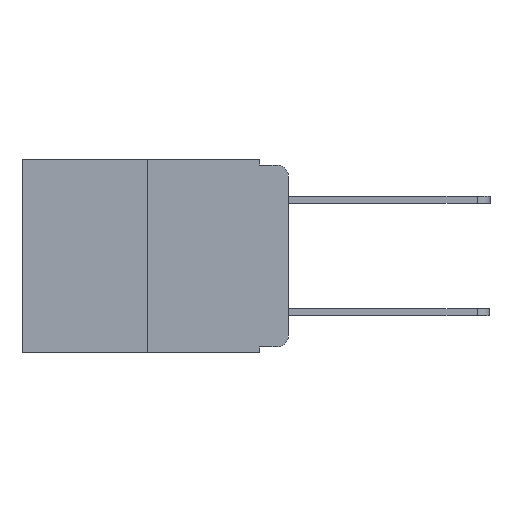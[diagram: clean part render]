
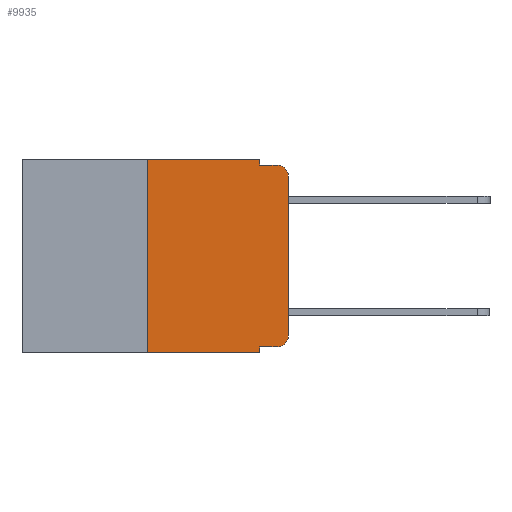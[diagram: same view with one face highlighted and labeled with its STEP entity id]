
A CAD part, left-side view. The second image highlights one B-rep face of the part: STEP entity #9935.
In plain terms, the highlighted planar face has unit normal (-1, 0, 0).
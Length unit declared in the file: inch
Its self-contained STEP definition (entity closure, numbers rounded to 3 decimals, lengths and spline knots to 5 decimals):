
#72 = DIRECTION ( 'NONE',  ( 0., 0., -1. ) ) ;
#94 = CARTESIAN_POINT ( 'NONE',  ( 0., 0.051, 0. ) ) ;
#124 = VECTOR ( 'NONE', #6096, 39.37008 ) ;
#268 = LINE ( 'NONE', #14664, #12533 ) ;
#565 = VERTEX_POINT ( 'NONE', #94 ) ;
#668 = ORIENTED_EDGE ( 'NONE', *, *, #2061, .T. ) ;
#820 = ORIENTED_EDGE ( 'NONE', *, *, #12431, .F. ) ;
#884 = VECTOR ( 'NONE', #6297, 39.37008 ) ;
#1126 = CARTESIAN_POINT ( 'NONE',  ( 0., 0.473, 0. ) ) ;
#1219 = PLANE ( 'NONE',  #7484 ) ;
#1458 = VERTEX_POINT ( 'NONE', #3909 ) ;
#1561 = DIRECTION ( 'NONE',  ( -1., 0., 0. ) ) ;
#1627 = ORIENTED_EDGE ( 'NONE', *, *, #7984, .T. ) ;
#1894 = ORIENTED_EDGE ( 'NONE', *, *, #3632, .F. ) ;
#2044 = VECTOR ( 'NONE', #5816, 39.37008 ) ;
#2061 = EDGE_CURVE ( 'NONE', #7726, #11921, #12033, .T. ) ;
#2075 = VERTEX_POINT ( 'NONE', #14688 ) ;
#2079 = CARTESIAN_POINT ( 'NONE',  ( 0., 0.25, 0. ) ) ;
#2183 = LINE ( 'NONE', #4996, #5178 ) ;
#2314 = VERTEX_POINT ( 'NONE', #8656 ) ;
#2509 = LINE ( 'NONE', #5091, #8574 ) ;
#2511 = CARTESIAN_POINT ( 'NONE',  ( 0., 0.473, 0. ) ) ;
#2585 = DIRECTION ( 'NONE',  ( 0., -1., 0. ) ) ;
#2598 = ORIENTED_EDGE ( 'NONE', *, *, #6688, .T. ) ;
#3262 = CARTESIAN_POINT ( 'NONE',  ( 0., 0.051, -0.333 ) ) ;
#3414 = LINE ( 'NONE', #4398, #8611 ) ;
#3632 = EDGE_CURVE ( 'NONE', #1458, #3977, #4687, .T. ) ;
#3762 = VERTEX_POINT ( 'NONE', #7849 ) ;
#3842 = DIRECTION ( 'NONE',  ( 1., 0., 0. ) ) ;
#3892 = EDGE_LOOP ( 'NONE', ( #1627, #8712, #4484, #820, #11541, #1894, #6085, #6919, #668, #2598 ) ) ;
#3909 = CARTESIAN_POINT ( 'NONE',  ( 0., 0.25, -0.343 ) ) ;
#3977 = VERTEX_POINT ( 'NONE', #2079 ) ;
#4398 = CARTESIAN_POINT ( 'NONE',  ( 0., 0., 0. ) ) ;
#4484 = ORIENTED_EDGE ( 'NONE', *, *, #13421, .F. ) ;
#4687 = LINE ( 'NONE', #13115, #884 ) ;
#4996 = CARTESIAN_POINT ( 'NONE',  ( 0., 0.051, 0. ) ) ;
#5091 = CARTESIAN_POINT ( 'NONE',  ( 0., 0.473, -0.343 ) ) ;
#5178 = VECTOR ( 'NONE', #10777, 39.37008 ) ;
#5816 = DIRECTION ( 'NONE',  ( 0., -1., 0. ) ) ;
#5832 = EDGE_CURVE ( 'NONE', #2314, #13918, #6987, .T. ) ;
#6019 = CARTESIAN_POINT ( 'NONE',  ( 0., 0.051, -0.333 ) ) ;
#6085 = ORIENTED_EDGE ( 'NONE', *, *, #9285, .T. ) ;
#6096 = DIRECTION ( 'NONE',  ( 0., -1., 0. ) ) ;
#6297 = DIRECTION ( 'NONE',  ( 0., 0., 1. ) ) ;
#6489 = EDGE_CURVE ( 'NONE', #7726, #2075, #2183, .T. ) ;
#6688 = EDGE_CURVE ( 'NONE', #11921, #3762, #8808, .T. ) ;
#6919 = ORIENTED_EDGE ( 'NONE', *, *, #6489, .F. ) ;
#6987 = CIRCLE ( 'NONE', #12227, 0.02 ) ;
#7406 = DIRECTION ( 'NONE',  ( -1., 0., 0. ) ) ;
#7484 = AXIS2_PLACEMENT_3D ( 'NONE', #2511, #3842, #11955 ) ;
#7726 = VERTEX_POINT ( 'NONE', #6019 ) ;
#7849 = CARTESIAN_POINT ( 'NONE',  ( 0., 0., -0.313 ) ) ;
#7984 = EDGE_CURVE ( 'NONE', #3762, #2314, #3414, .T. ) ;
#8574 = VECTOR ( 'NONE', #2585, 39.37008 ) ;
#8611 = VECTOR ( 'NONE', #10234, 39.37008 ) ;
#8656 = CARTESIAN_POINT ( 'NONE',  ( 0., 0., -0.03 ) ) ;
#8712 = ORIENTED_EDGE ( 'NONE', *, *, #5832, .T. ) ;
#8808 = CIRCLE ( 'NONE', #14838, 0.02 ) ;
#8850 = CARTESIAN_POINT ( 'NONE',  ( 0., 0.02, -0.313 ) ) ;
#9285 = EDGE_CURVE ( 'NONE', #1458, #2075, #2509, .T. ) ;
#9424 = VECTOR ( 'NONE', #10326, 39.37008 ) ;
#9473 = FACE_OUTER_BOUND ( 'NONE', #3892, .T. ) ;
#9599 = CARTESIAN_POINT ( 'NONE',  ( 0., 0.051, -0.01 ) ) ;
#9935 = ADVANCED_FACE ( 'NONE', ( #9473 ), #1219, .F. ) ;
#10017 = DIRECTION ( 'NONE',  ( 0., 0., -1. ) ) ;
#10234 = DIRECTION ( 'NONE',  ( 0., 0., 1. ) ) ;
#10326 = DIRECTION ( 'NONE',  ( 0., -1., 0. ) ) ;
#10777 = DIRECTION ( 'NONE',  ( 0., 0., -1. ) ) ;
#11270 = EDGE_CURVE ( 'NONE', #3977, #565, #12730, .T. ) ;
#11477 = DIRECTION ( 'NONE',  ( 0., 0., -1. ) ) ;
#11541 = ORIENTED_EDGE ( 'NONE', *, *, #11270, .F. ) ;
#11921 = VERTEX_POINT ( 'NONE', #15056 ) ;
#11955 = DIRECTION ( 'NONE',  ( 0., 0., -1. ) ) ;
#12033 = LINE ( 'NONE', #3262, #9424 ) ;
#12227 = AXIS2_PLACEMENT_3D ( 'NONE', #14117, #7406, #72 ) ;
#12431 = EDGE_CURVE ( 'NONE', #565, #13571, #268, .T. ) ;
#12533 = VECTOR ( 'NONE', #11477, 39.37008 ) ;
#12730 = LINE ( 'NONE', #1126, #124 ) ;
#13058 = CARTESIAN_POINT ( 'NONE',  ( 0., 0.051, -0.01 ) ) ;
#13115 = CARTESIAN_POINT ( 'NONE',  ( 0., 0.25, 0. ) ) ;
#13421 = EDGE_CURVE ( 'NONE', #13571, #13918, #14387, .T. ) ;
#13466 = CARTESIAN_POINT ( 'NONE',  ( 0., 0.02, -0.01 ) ) ;
#13571 = VERTEX_POINT ( 'NONE', #9599 ) ;
#13918 = VERTEX_POINT ( 'NONE', #13466 ) ;
#14117 = CARTESIAN_POINT ( 'NONE',  ( 0., 0.02, -0.03 ) ) ;
#14387 = LINE ( 'NONE', #13058, #2044 ) ;
#14664 = CARTESIAN_POINT ( 'NONE',  ( 0., 0.051, 0. ) ) ;
#14688 = CARTESIAN_POINT ( 'NONE',  ( 0., 0.051, -0.343 ) ) ;
#14838 = AXIS2_PLACEMENT_3D ( 'NONE', #8850, #1561, #10017 ) ;
#15056 = CARTESIAN_POINT ( 'NONE',  ( 0., 0.02, -0.333 ) ) ;
